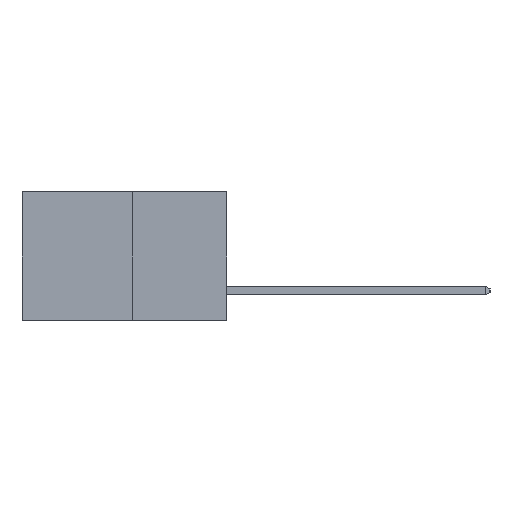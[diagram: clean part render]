
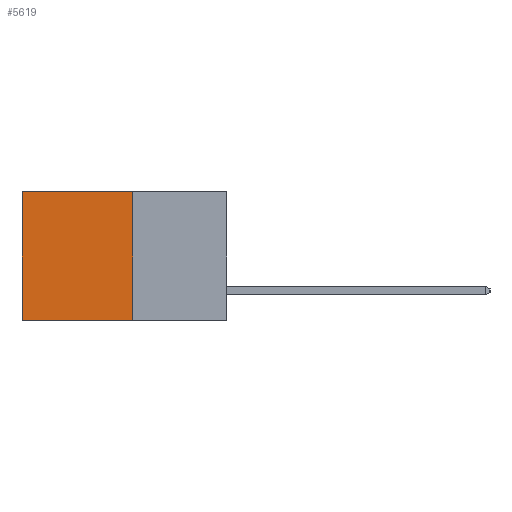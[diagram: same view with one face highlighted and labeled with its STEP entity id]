
A CAD part, left-side view. The second image highlights one B-rep face of the part: STEP entity #5619.
In plain terms, the highlighted planar face has unit normal (-1, 0, 0).
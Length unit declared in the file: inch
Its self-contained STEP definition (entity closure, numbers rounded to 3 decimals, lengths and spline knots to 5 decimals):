
#444 = CARTESIAN_POINT ( 'NONE',  ( 0.277, 0.59, 0. ) ) ;
#709 = FACE_OUTER_BOUND ( 'NONE', #5231, .T. ) ;
#821 = DIRECTION ( 'NONE',  ( 0., 0., -1. ) ) ;
#1184 = VECTOR ( 'NONE', #9434, 39.37008 ) ;
#1482 = CARTESIAN_POINT ( 'NONE',  ( 0.277, 0.27, -0.37 ) ) ;
#1627 = EDGE_CURVE ( 'NONE', #6927, #2923, #3845, .T. ) ;
#1973 = VECTOR ( 'NONE', #9659, 39.37008 ) ;
#2127 = ORIENTED_EDGE ( 'NONE', *, *, #5698, .T. ) ;
#2549 = PLANE ( 'NONE',  #9870 ) ;
#2923 = VERTEX_POINT ( 'NONE', #9538 ) ;
#3021 = DIRECTION ( 'NONE',  ( 0., 1., 0. ) ) ;
#3149 = VERTEX_POINT ( 'NONE', #6875 ) ;
#3331 = ORIENTED_EDGE ( 'NONE', *, *, #1627, .F. ) ;
#3416 = EDGE_CURVE ( 'NONE', #2923, #3149, #3514, .T. ) ;
#3514 = LINE ( 'NONE', #8332, #1184 ) ;
#3554 = CARTESIAN_POINT ( 'NONE',  ( 0.277, 0.59, -0.37 ) ) ;
#3845 = LINE ( 'NONE', #1482, #6204 ) ;
#4339 = CARTESIAN_POINT ( 'NONE',  ( 0.277, 0.27, 0. ) ) ;
#4368 = CARTESIAN_POINT ( 'NONE',  ( 0.277, 0.27, -0.37 ) ) ;
#5231 = EDGE_LOOP ( 'NONE', ( #2127, #5664, #3331, #10888 ) ) ;
#5619 = ADVANCED_FACE ( 'NONE', ( #709 ), #2549, .F. ) ;
#5664 = ORIENTED_EDGE ( 'NONE', *, *, #3416, .F. ) ;
#5698 = EDGE_CURVE ( 'NONE', #9366, #3149, #8973, .T. ) ;
#6121 = DIRECTION ( 'NONE',  ( 1., 0., 0. ) ) ;
#6204 = VECTOR ( 'NONE', #10685, 39.37008 ) ;
#6634 = LINE ( 'NONE', #10905, #8662 ) ;
#6875 = CARTESIAN_POINT ( 'NONE',  ( 0.277, 0.59, -0.37 ) ) ;
#6927 = VERTEX_POINT ( 'NONE', #4339 ) ;
#7807 = EDGE_CURVE ( 'NONE', #6927, #9366, #6634, .T. ) ;
#8332 = CARTESIAN_POINT ( 'NONE',  ( 0.277, 0.27, -0.37 ) ) ;
#8662 = VECTOR ( 'NONE', #3021, 39.37008 ) ;
#8973 = LINE ( 'NONE', #3554, #1973 ) ;
#9366 = VERTEX_POINT ( 'NONE', #444 ) ;
#9434 = DIRECTION ( 'NONE',  ( 0., 1., 0. ) ) ;
#9538 = CARTESIAN_POINT ( 'NONE',  ( 0.277, 0.27, -0.37 ) ) ;
#9659 = DIRECTION ( 'NONE',  ( 0., 0., -1. ) ) ;
#9870 = AXIS2_PLACEMENT_3D ( 'NONE', #4368, #6121, #821 ) ;
#10685 = DIRECTION ( 'NONE',  ( 0., 0., -1. ) ) ;
#10888 = ORIENTED_EDGE ( 'NONE', *, *, #7807, .T. ) ;
#10905 = CARTESIAN_POINT ( 'NONE',  ( 0.277, 0.27, 0. ) ) ;
